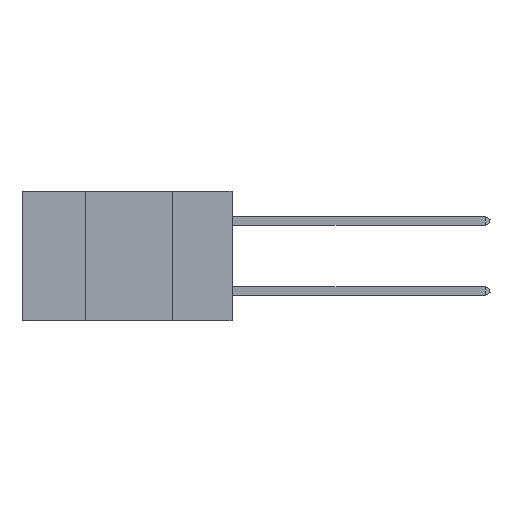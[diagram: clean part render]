
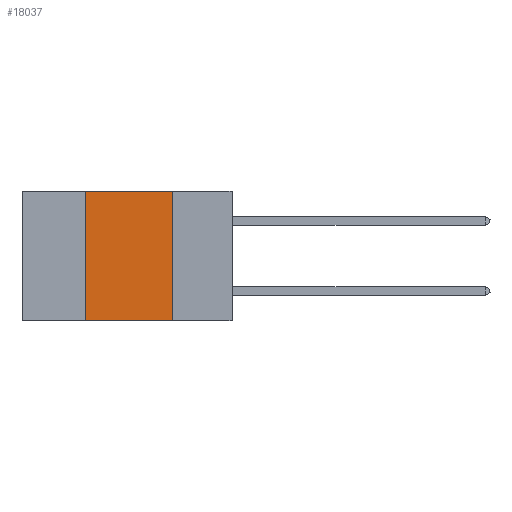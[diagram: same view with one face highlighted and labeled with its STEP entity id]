
A CAD part, left-side view. The second image highlights one B-rep face of the part: STEP entity #18037.
In plain terms, the highlighted planar face has unit normal (-1, 0, 0).
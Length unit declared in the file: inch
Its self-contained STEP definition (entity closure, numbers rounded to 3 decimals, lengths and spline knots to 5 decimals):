
#756 = VECTOR ( 'NONE', #14951, 39.37008 ) ;
#910 = DIRECTION ( 'NONE',  ( 0., 0., -1. ) ) ;
#1134 = VERTEX_POINT ( 'NONE', #41778 ) ;
#1808 = EDGE_CURVE ( 'NONE', #43066, #8780, #28027, .T. ) ;
#3469 = ORIENTED_EDGE ( 'NONE', *, *, #7640, .F. ) ;
#5489 = CARTESIAN_POINT ( 'NONE',  ( 0., 0.42, -0.37 ) ) ;
#7640 = EDGE_CURVE ( 'NONE', #27216, #1134, #31855, .T. ) ;
#8780 = VERTEX_POINT ( 'NONE', #18613 ) ;
#13053 = LINE ( 'NONE', #41013, #29101 ) ;
#13531 = EDGE_CURVE ( 'NONE', #43066, #1134, #45406, .T. ) ;
#14951 = DIRECTION ( 'NONE',  ( 0., -1., 0. ) ) ;
#15771 = ORIENTED_EDGE ( 'NONE', *, *, #13531, .T. ) ;
#15863 = CARTESIAN_POINT ( 'NONE',  ( 0., 0.6, 0. ) ) ;
#18037 = ADVANCED_FACE ( 'NONE', ( #31323 ), #18680, .F. ) ;
#18094 = ORIENTED_EDGE ( 'NONE', *, *, #44904, .F. ) ;
#18613 = CARTESIAN_POINT ( 'NONE',  ( 0., 0.42, 0. ) ) ;
#18680 = PLANE ( 'NONE',  #41004 ) ;
#19852 = DIRECTION ( 'NONE',  ( 1., 0., 0. ) ) ;
#23361 = DIRECTION ( 'NONE',  ( 0., 0., -1. ) ) ;
#26809 = ORIENTED_EDGE ( 'NONE', *, *, #1808, .F. ) ;
#27216 = VERTEX_POINT ( 'NONE', #43680 ) ;
#28027 = LINE ( 'NONE', #41772, #34590 ) ;
#29101 = VECTOR ( 'NONE', #36533, 39.37008 ) ;
#31323 = FACE_OUTER_BOUND ( 'NONE', #42416, .T. ) ;
#31855 = LINE ( 'NONE', #38483, #47910 ) ;
#34590 = VECTOR ( 'NONE', #45725, 39.37008 ) ;
#36533 = DIRECTION ( 'NONE',  ( 0., -1., 0. ) ) ;
#37729 = CARTESIAN_POINT ( 'NONE',  ( 0., 0.6, -0.37 ) ) ;
#38483 = CARTESIAN_POINT ( 'NONE',  ( 0., 0.17, 0. ) ) ;
#41004 = AXIS2_PLACEMENT_3D ( 'NONE', #15863, #19852, #910 ) ;
#41013 = CARTESIAN_POINT ( 'NONE',  ( 0., 0.6, 0. ) ) ;
#41772 = CARTESIAN_POINT ( 'NONE',  ( 0., 0.42, 0. ) ) ;
#41778 = CARTESIAN_POINT ( 'NONE',  ( 0., 0.17, -0.37 ) ) ;
#42416 = EDGE_LOOP ( 'NONE', ( #3469, #18094, #26809, #15771 ) ) ;
#43066 = VERTEX_POINT ( 'NONE', #5489 ) ;
#43680 = CARTESIAN_POINT ( 'NONE',  ( 0., 0.17, 0. ) ) ;
#44904 = EDGE_CURVE ( 'NONE', #8780, #27216, #13053, .T. ) ;
#45406 = LINE ( 'NONE', #37729, #756 ) ;
#45725 = DIRECTION ( 'NONE',  ( 0., 0., 1. ) ) ;
#47910 = VECTOR ( 'NONE', #23361, 39.37008 ) ;
